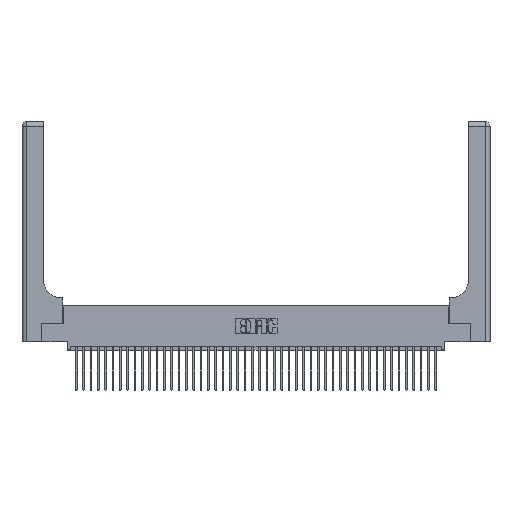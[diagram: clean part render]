
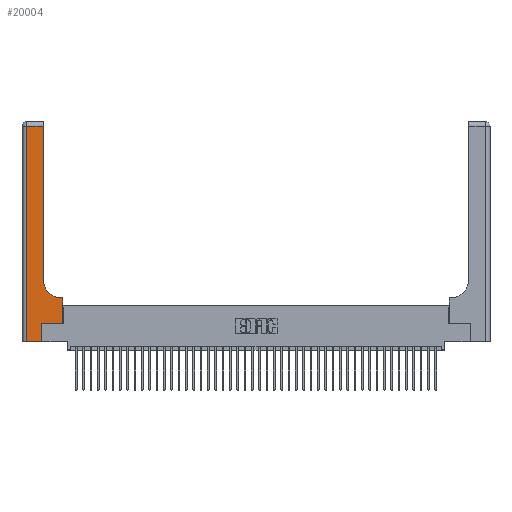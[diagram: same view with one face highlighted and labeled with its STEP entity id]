
A CAD part, top view. The second image highlights one B-rep face of the part: STEP entity #20004.
In plain terms, the highlighted planar face has unit normal (0, 0, 1).
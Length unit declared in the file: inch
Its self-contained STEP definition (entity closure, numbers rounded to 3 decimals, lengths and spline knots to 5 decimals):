
#755 = DIRECTION ( 'NONE',  ( 0., 1., 0. ) ) ;
#1241 = CARTESIAN_POINT ( 'NONE',  ( 0.269, 0.25, 0.37 ) ) ;
#1535 = PLANE ( 'NONE',  #21732 ) ;
#2211 = VERTEX_POINT ( 'NONE', #20935 ) ;
#2256 = DIRECTION ( 'NONE',  ( -1., 0., 0. ) ) ;
#2657 = VERTEX_POINT ( 'NONE', #37179 ) ;
#2758 = CARTESIAN_POINT ( 'NONE',  ( 0.5585, 0.25, 0.37 ) ) ;
#2867 = VECTOR ( 'NONE', #755, 39.37008 ) ;
#3075 = FACE_OUTER_BOUND ( 'NONE', #18871, .T. ) ;
#3102 = CARTESIAN_POINT ( 'NONE',  ( 0.2915, 2.94, 0.37 ) ) ;
#4487 = LINE ( 'NONE', #19099, #13382 ) ;
#4528 = VERTEX_POINT ( 'NONE', #29165 ) ;
#5120 = LINE ( 'NONE', #16909, #30857 ) ;
#5837 = CARTESIAN_POINT ( 'NONE',  ( 0.06, 3., 0.37 ) ) ;
#6315 = LINE ( 'NONE', #5837, #40987 ) ;
#7203 = ORIENTED_EDGE ( 'NONE', *, *, #10568, .T. ) ;
#8312 = DIRECTION ( 'NONE',  ( 0., 0., -1. ) ) ;
#9180 = ORIENTED_EDGE ( 'NONE', *, *, #19820, .T. ) ;
#9397 = LINE ( 'NONE', #34320, #35149 ) ;
#9414 = EDGE_CURVE ( 'NONE', #20877, #24408, #5120, .T. ) ;
#9772 = CARTESIAN_POINT ( 'NONE',  ( 0.5585, 0.25, 0.37 ) ) ;
#10568 = EDGE_CURVE ( 'NONE', #2211, #38209, #4487, .T. ) ;
#10760 = LINE ( 'NONE', #13966, #2867 ) ;
#11329 = VERTEX_POINT ( 'NONE', #2758 ) ;
#12354 = DIRECTION ( 'NONE',  ( 1., 0., 0. ) ) ;
#13118 = DIRECTION ( 'NONE',  ( 0., 1., 0. ) ) ;
#13382 = VECTOR ( 'NONE', #12354, 39.37008 ) ;
#13877 = CARTESIAN_POINT ( 'NONE',  ( 0.269, 0., 0.37 ) ) ;
#13966 = CARTESIAN_POINT ( 'NONE',  ( 0.269, 0., 0.37 ) ) ;
#14142 = CARTESIAN_POINT ( 'NONE',  ( 0.5585, 0.6, 0.37 ) ) ;
#15825 = CARTESIAN_POINT ( 'NONE',  ( 0.5415, 0.85, 0.37 ) ) ;
#16909 = CARTESIAN_POINT ( 'NONE',  ( 0., 2.94, 0.37 ) ) ;
#17568 = DIRECTION ( 'NONE',  ( 0., 1., 0. ) ) ;
#17599 = ORIENTED_EDGE ( 'NONE', *, *, #9414, .T. ) ;
#18443 = EDGE_CURVE ( 'NONE', #11329, #18723, #21745, .T. ) ;
#18542 = DIRECTION ( 'NONE',  ( 0., -1., 0. ) ) ;
#18723 = VERTEX_POINT ( 'NONE', #14142 ) ;
#18777 = LINE ( 'NONE', #22401, #27744 ) ;
#18871 = EDGE_LOOP ( 'NONE', ( #9180, #17599, #27127, #7203, #29829, #31428, #23541, #34586, #28820 ) ) ;
#19099 = CARTESIAN_POINT ( 'NONE',  ( 0., 0., 0.37 ) ) ;
#19181 = DIRECTION ( 'NONE',  ( 1., 0., 0. ) ) ;
#19485 = EDGE_CURVE ( 'NONE', #29477, #2657, #32143, .T. ) ;
#19820 = EDGE_CURVE ( 'NONE', #2657, #20877, #9397, .T. ) ;
#19902 = EDGE_CURVE ( 'NONE', #4528, #11329, #43010, .T. ) ;
#20004 = ADVANCED_FACE ( 'NONE', ( #3075 ), #1535, .F. ) ;
#20877 = VERTEX_POINT ( 'NONE', #3102 ) ;
#20935 = CARTESIAN_POINT ( 'NONE',  ( 0.06, 0., 0.37 ) ) ;
#21732 = AXIS2_PLACEMENT_3D ( 'NONE', #28444, #8312, #31811 ) ;
#21745 = LINE ( 'NONE', #9772, #27529 ) ;
#22401 = CARTESIAN_POINT ( 'NONE',  ( 0.2915, 0.6, 0.37 ) ) ;
#23058 = VECTOR ( 'NONE', #38136, 39.37008 ) ;
#23541 = ORIENTED_EDGE ( 'NONE', *, *, #18443, .T. ) ;
#24408 = VERTEX_POINT ( 'NONE', #41801 ) ;
#27127 = ORIENTED_EDGE ( 'NONE', *, *, #39759, .T. ) ;
#27529 = VECTOR ( 'NONE', #13118, 39.37008 ) ;
#27744 = VECTOR ( 'NONE', #2256, 39.37008 ) ;
#28444 = CARTESIAN_POINT ( 'NONE',  ( 0., 3., 0.37 ) ) ;
#28820 = ORIENTED_EDGE ( 'NONE', *, *, #19485, .T. ) ;
#29165 = CARTESIAN_POINT ( 'NONE',  ( 0.269, 0.25, 0.37 ) ) ;
#29477 = VERTEX_POINT ( 'NONE', #35499 ) ;
#29829 = ORIENTED_EDGE ( 'NONE', *, *, #38933, .T. ) ;
#30857 = VECTOR ( 'NONE', #33808, 39.37008 ) ;
#31428 = ORIENTED_EDGE ( 'NONE', *, *, #19902, .T. ) ;
#31811 = DIRECTION ( 'NONE',  ( -1., 0., 0. ) ) ;
#32143 = CIRCLE ( 'NONE', #32406, 0.25 ) ;
#32406 = AXIS2_PLACEMENT_3D ( 'NONE', #15825, #39319, #19181 ) ;
#33808 = DIRECTION ( 'NONE',  ( -1., 0., 0. ) ) ;
#34320 = CARTESIAN_POINT ( 'NONE',  ( 0.2915, 3., 0.37 ) ) ;
#34586 = ORIENTED_EDGE ( 'NONE', *, *, #36260, .T. ) ;
#35149 = VECTOR ( 'NONE', #17568, 39.37008 ) ;
#35499 = CARTESIAN_POINT ( 'NONE',  ( 0.5415, 0.6, 0.37 ) ) ;
#36260 = EDGE_CURVE ( 'NONE', #18723, #29477, #18777, .T. ) ;
#37179 = CARTESIAN_POINT ( 'NONE',  ( 0.2915, 0.85, 0.37 ) ) ;
#38136 = DIRECTION ( 'NONE',  ( 1., 0., 0. ) ) ;
#38209 = VERTEX_POINT ( 'NONE', #13877 ) ;
#38933 = EDGE_CURVE ( 'NONE', #38209, #4528, #10760, .T. ) ;
#39319 = DIRECTION ( 'NONE',  ( 0., 0., -1. ) ) ;
#39759 = EDGE_CURVE ( 'NONE', #24408, #2211, #6315, .T. ) ;
#40987 = VECTOR ( 'NONE', #18542, 39.37008 ) ;
#41801 = CARTESIAN_POINT ( 'NONE',  ( 0.06, 2.94, 0.37 ) ) ;
#43010 = LINE ( 'NONE', #1241, #23058 ) ;
